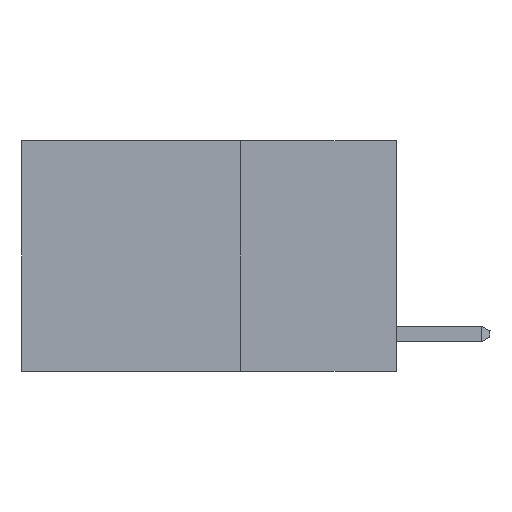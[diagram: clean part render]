
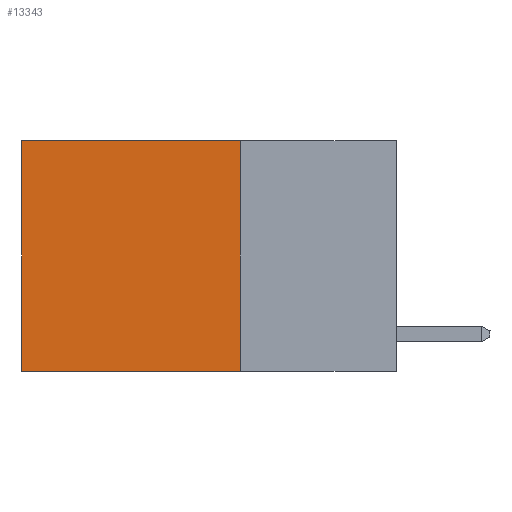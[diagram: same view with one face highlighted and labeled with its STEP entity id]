
A CAD part, left-side view. The second image highlights one B-rep face of the part: STEP entity #13343.
In plain terms, the highlighted planar face has unit normal (-1, 0, 0).
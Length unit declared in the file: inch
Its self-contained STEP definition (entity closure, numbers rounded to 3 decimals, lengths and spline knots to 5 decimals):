
#46 = DIRECTION ( 'NONE',  ( 0., 0., -1. ) ) ;
#75 = CARTESIAN_POINT ( 'NONE',  ( 0.2625, 0.6, 0. ) ) ;
#1233 = EDGE_CURVE ( 'NONE', #9063, #12295, #3914, .T. ) ;
#1618 = CARTESIAN_POINT ( 'NONE',  ( 0.2625, 0.6, -0.37 ) ) ;
#2413 = LINE ( 'NONE', #8397, #17023 ) ;
#3598 = EDGE_CURVE ( 'NONE', #4448, #9063, #11382, .T. ) ;
#3914 = LINE ( 'NONE', #9339, #11949 ) ;
#4146 = DIRECTION ( 'NONE',  ( 1., 0., 0. ) ) ;
#4236 = FACE_OUTER_BOUND ( 'NONE', #4516, .T. ) ;
#4448 = VERTEX_POINT ( 'NONE', #6168 ) ;
#4516 = EDGE_LOOP ( 'NONE', ( #9032, #13394, #15096, #10939 ) ) ;
#4608 = DIRECTION ( 'NONE',  ( 0., 0., -1. ) ) ;
#6168 = CARTESIAN_POINT ( 'NONE',  ( 0.2625, 0.25, 0. ) ) ;
#7399 = LINE ( 'NONE', #75, #7601 ) ;
#7601 = VECTOR ( 'NONE', #8917, 39.37008 ) ;
#7775 = CARTESIAN_POINT ( 'NONE',  ( 0.2625, 0.6, 0. ) ) ;
#8110 = DIRECTION ( 'NONE',  ( 0., 1., 0. ) ) ;
#8167 = AXIS2_PLACEMENT_3D ( 'NONE', #17141, #4146, #46 ) ;
#8397 = CARTESIAN_POINT ( 'NONE',  ( 0.2625, 0.25, 0. ) ) ;
#8917 = DIRECTION ( 'NONE',  ( 0., 0., -1. ) ) ;
#9032 = ORIENTED_EDGE ( 'NONE', *, *, #17528, .T. ) ;
#9063 = VERTEX_POINT ( 'NONE', #14433 ) ;
#9191 = VERTEX_POINT ( 'NONE', #7775 ) ;
#9339 = CARTESIAN_POINT ( 'NONE',  ( 0.2625, 0.25, -0.37 ) ) ;
#10939 = ORIENTED_EDGE ( 'NONE', *, *, #18672, .T. ) ;
#11382 = LINE ( 'NONE', #17154, #13452 ) ;
#11949 = VECTOR ( 'NONE', #18129, 39.37008 ) ;
#12295 = VERTEX_POINT ( 'NONE', #1618 ) ;
#13343 = ADVANCED_FACE ( 'NONE', ( #4236 ), #18729, .F. ) ;
#13394 = ORIENTED_EDGE ( 'NONE', *, *, #1233, .F. ) ;
#13452 = VECTOR ( 'NONE', #4608, 39.37008 ) ;
#14433 = CARTESIAN_POINT ( 'NONE',  ( 0.2625, 0.25, -0.37 ) ) ;
#15096 = ORIENTED_EDGE ( 'NONE', *, *, #3598, .F. ) ;
#17023 = VECTOR ( 'NONE', #8110, 39.37008 ) ;
#17141 = CARTESIAN_POINT ( 'NONE',  ( 0.2625, 0.25, 0. ) ) ;
#17154 = CARTESIAN_POINT ( 'NONE',  ( 0.2625, 0.25, 0. ) ) ;
#17528 = EDGE_CURVE ( 'NONE', #9191, #12295, #7399, .T. ) ;
#18129 = DIRECTION ( 'NONE',  ( 0., 1., 0. ) ) ;
#18672 = EDGE_CURVE ( 'NONE', #4448, #9191, #2413, .T. ) ;
#18729 = PLANE ( 'NONE',  #8167 ) ;
